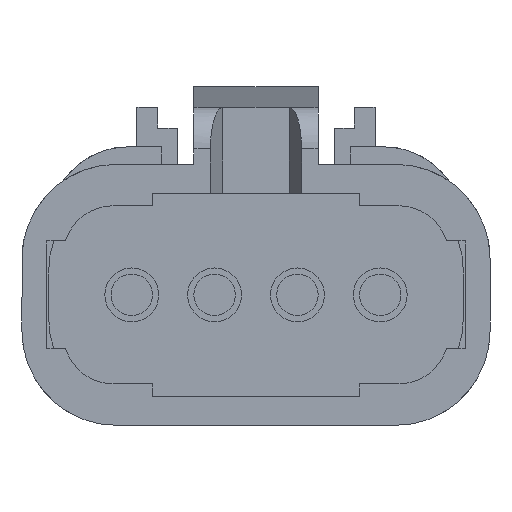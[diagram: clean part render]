
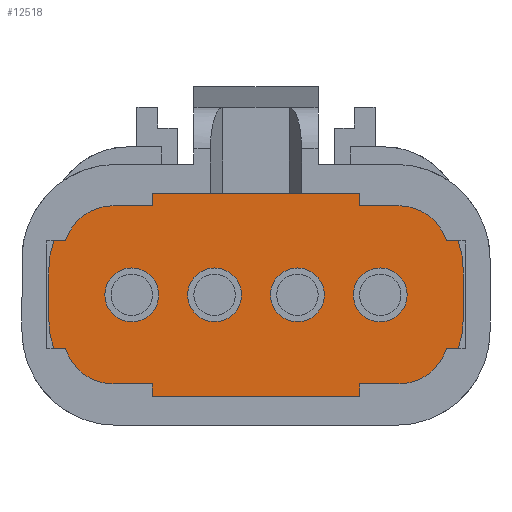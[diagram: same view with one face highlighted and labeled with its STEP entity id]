
A CAD part, front view. The second image highlights one B-rep face of the part: STEP entity #12518.
In plain terms, the highlighted planar face has unit normal (0, -1, 0).
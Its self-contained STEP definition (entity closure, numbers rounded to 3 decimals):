
#31 = CARTESIAN_POINT ( 'NONE',  ( 9.277, 0.032, 11.722 ) ) ;
#158 = DIRECTION ( 'NONE',  ( 0., -1., 0. ) ) ;
#267 = EDGE_CURVE ( 'NONE', #3505, #3678, #8905, .T. ) ;
#401 = DIRECTION ( 'NONE',  ( 0., 1., 0. ) ) ;
#629 = CIRCLE ( 'NONE', #10572, 0.65 ) ;
#683 = DIRECTION ( 'NONE',  ( 0., 0., 1. ) ) ;
#842 = EDGE_CURVE ( 'NONE', #3943, #9786, #10768, .T. ) ;
#934 = DIRECTION ( 'NONE',  ( -1., 0., 0. ) ) ;
#954 = CARTESIAN_POINT ( 'NONE',  ( 7.477, 0.032, 9.922 ) ) ;
#969 = LINE ( 'NONE', #7506, #8911 ) ;
#1073 = ORIENTED_EDGE ( 'NONE', *, *, #6733, .F. ) ;
#1563 = CARTESIAN_POINT ( 'NONE',  ( 3.927, 0.032, 12.372 ) ) ;
#1584 = CARTESIAN_POINT ( 'NONE',  ( -0.723, 0.032, 13.022 ) ) ;
#1592 = LINE ( 'NONE', #7227, #12161 ) ;
#1626 = FACE_OUTER_BOUND ( 'NONE', #8329, .T. ) ;
#1644 = CARTESIAN_POINT ( 'NONE',  ( 4.627, 0.032, 12.372 ) ) ;
#1683 = CARTESIAN_POINT ( 'NONE',  ( 1.077, 0.032, 13.022 ) ) ;
#1760 = CARTESIAN_POINT ( 'NONE',  ( 9.277, 0.032, 13.022 ) ) ;
#1831 = AXIS2_PLACEMENT_3D ( 'NONE', #9878, #13264, #3116 ) ;
#1903 = CARTESIAN_POINT ( 'NONE',  ( 0.627, 0.032, 12.372 ) ) ;
#1943 = CIRCLE ( 'NONE', #8327, 0.65 ) ;
#2380 = DIRECTION ( 'NONE',  ( -1., 0., 0. ) ) ;
#2409 = CARTESIAN_POINT ( 'NONE',  ( 7.277, 0.032, 12.372 ) ) ;
#2475 = EDGE_CURVE ( 'NONE', #8021, #3505, #8771, .T. ) ;
#2527 = EDGE_CURVE ( 'NONE', #9786, #3943, #1943, .T. ) ;
#2537 = CARTESIAN_POINT ( 'NONE',  ( 1.277, 0.032, 12.372 ) ) ;
#2554 = DIRECTION ( 'NONE',  ( -1., 0., 0. ) ) ;
#2583 = ORIENTED_EDGE ( 'NONE', *, *, #10625, .F. ) ;
#2644 = DIRECTION ( 'NONE',  ( -1., 0., 0. ) ) ;
#2749 = AXIS2_PLACEMENT_3D ( 'NONE', #13836, #8362, #7032 ) ;
#2914 = EDGE_CURVE ( 'NONE', #12138, #14171, #9163, .T. ) ;
#3116 = DIRECTION ( 'NONE',  ( -1., 0., 0. ) ) ;
#3173 = EDGE_CURVE ( 'NONE', #10151, #12673, #629, .T. ) ;
#3254 = AXIS2_PLACEMENT_3D ( 'NONE', #13728, #158, #13521 ) ;
#3291 = DIRECTION ( 'NONE',  ( 0., 0., -1. ) ) ;
#3296 = ORIENTED_EDGE ( 'NONE', *, *, #8671, .F. ) ;
#3456 = EDGE_CURVE ( 'NONE', #5921, #8046, #9171, .T. ) ;
#3505 = VERTEX_POINT ( 'NONE', #1584 ) ;
#3531 = DIRECTION ( 'NONE',  ( 1., 0., 0. ) ) ;
#3569 = DIRECTION ( 'NONE',  ( 0., -1., 0. ) ) ;
#3678 = VERTEX_POINT ( 'NONE', #6551 ) ;
#3943 = VERTEX_POINT ( 'NONE', #1563 ) ;
#4055 = VECTOR ( 'NONE', #683, 1000. ) ;
#4157 = FACE_BOUND ( 'NONE', #13364, .T. ) ;
#4186 = DIRECTION ( 'NONE',  ( 0., 1., 0. ) ) ;
#4331 = ORIENTED_EDGE ( 'NONE', *, *, #267, .F. ) ;
#4480 = CARTESIAN_POINT ( 'NONE',  ( 9.277, 0.032, 11.722 ) ) ;
#4681 = VERTEX_POINT ( 'NONE', #954 ) ;
#4792 = DIRECTION ( 'NONE',  ( 0., -1., 0. ) ) ;
#5004 = CARTESIAN_POINT ( 'NONE',  ( 7.477, 0.032, 11.722 ) ) ;
#5067 = ORIENTED_EDGE ( 'NONE', *, *, #2914, .F. ) ;
#5272 = EDGE_CURVE ( 'NONE', #4681, #8836, #969, .T. ) ;
#5325 = ORIENTED_EDGE ( 'NONE', *, *, #9541, .F. ) ;
#5363 = CIRCLE ( 'NONE', #2749, 0.65 ) ;
#5431 = CARTESIAN_POINT ( 'NONE',  ( 3.277, 0.032, 12.372 ) ) ;
#5501 = CARTESIAN_POINT ( 'NONE',  ( -0.723, 0.032, 11.722 ) ) ;
#5554 = EDGE_CURVE ( 'NONE', #14171, #12138, #5363, .T. ) ;
#5921 = VERTEX_POINT ( 'NONE', #11605 ) ;
#6033 = CARTESIAN_POINT ( 'NONE',  ( 1.927, 0.032, 12.372 ) ) ;
#6052 = AXIS2_PLACEMENT_3D ( 'NONE', #14604, #4186, #8924 ) ;
#6108 = CARTESIAN_POINT ( 'NONE',  ( 7.477, 0.032, 14.822 ) ) ;
#6206 = DIRECTION ( 'NONE',  ( 0., 1., 0. ) ) ;
#6244 = CIRCLE ( 'NONE', #9099, 0.65 ) ;
#6374 = FACE_BOUND ( 'NONE', #11573, .T. ) ;
#6500 = ORIENTED_EDGE ( 'NONE', *, *, #5272, .F. ) ;
#6551 = CARTESIAN_POINT ( 'NONE',  ( 1.077, 0.032, 14.822 ) ) ;
#6733 = EDGE_CURVE ( 'NONE', #8046, #5921, #6244, .T. ) ;
#6874 = AXIS2_PLACEMENT_3D ( 'NONE', #5004, #401, #14109 ) ;
#6899 = CARTESIAN_POINT ( 'NONE',  ( 3.277, 0.032, 12.372 ) ) ;
#6952 = CARTESIAN_POINT ( 'NONE',  ( 1.277, 0.032, 12.372 ) ) ;
#7032 = DIRECTION ( 'NONE',  ( -1., 0., 0. ) ) ;
#7153 = EDGE_CURVE ( 'NONE', #12673, #10151, #13356, .T. ) ;
#7222 = ORIENTED_EDGE ( 'NONE', *, *, #2527, .F. ) ;
#7227 = CARTESIAN_POINT ( 'NONE',  ( 7.477, 0.032, 14.822 ) ) ;
#7506 = CARTESIAN_POINT ( 'NONE',  ( 7.477, 0.032, 9.922 ) ) ;
#7743 = DIRECTION ( 'NONE',  ( -1., 0., 0. ) ) ;
#8021 = VERTEX_POINT ( 'NONE', #12366 ) ;
#8046 = VERTEX_POINT ( 'NONE', #12517 ) ;
#8293 = CIRCLE ( 'NONE', #10910, 1.8 ) ;
#8327 = AXIS2_PLACEMENT_3D ( 'NONE', #5431, #9967, #7743 ) ;
#8329 = EDGE_LOOP ( 'NONE', ( #3296, #6500, #12049, #2583, #5325, #14447, #4331, #14255 ) ) ;
#8362 = DIRECTION ( 'NONE',  ( 0., -1., 0. ) ) ;
#8407 = ORIENTED_EDGE ( 'NONE', *, *, #7153, .F. ) ;
#8579 = EDGE_LOOP ( 'NONE', ( #9759, #1073 ) ) ;
#8671 = EDGE_CURVE ( 'NONE', #8836, #8021, #12453, .T. ) ;
#8740 = DIRECTION ( 'NONE',  ( 0., 1., 0. ) ) ;
#8771 = LINE ( 'NONE', #5501, #4055 ) ;
#8836 = VERTEX_POINT ( 'NONE', #13852 ) ;
#8905 = CIRCLE ( 'NONE', #14339, 1.8 ) ;
#8911 = VECTOR ( 'NONE', #14444, 1000. ) ;
#8924 = DIRECTION ( 'NONE',  ( 1., 0., 0. ) ) ;
#9099 = AXIS2_PLACEMENT_3D ( 'NONE', #2409, #10275, #2554 ) ;
#9163 = CIRCLE ( 'NONE', #1831, 0.65 ) ;
#9171 = CIRCLE ( 'NONE', #3254, 0.65 ) ;
#9366 = DIRECTION ( 'NONE',  ( 0., -1., 0. ) ) ;
#9523 = DIRECTION ( 'NONE',  ( 1., 0., 0. ) ) ;
#9541 = EDGE_CURVE ( 'NONE', #14196, #11252, #8293, .T. ) ;
#9659 = VERTEX_POINT ( 'NONE', #31 ) ;
#9723 = EDGE_CURVE ( 'NONE', #9659, #4681, #12090, .T. ) ;
#9759 = ORIENTED_EDGE ( 'NONE', *, *, #3456, .F. ) ;
#9786 = VERTEX_POINT ( 'NONE', #12933 ) ;
#9878 = CARTESIAN_POINT ( 'NONE',  ( 5.277, 0.032, 12.372 ) ) ;
#9967 = DIRECTION ( 'NONE',  ( 0., -1., 0. ) ) ;
#10151 = VERTEX_POINT ( 'NONE', #1903 ) ;
#10275 = DIRECTION ( 'NONE',  ( 0., -1., 0. ) ) ;
#10572 = AXIS2_PLACEMENT_3D ( 'NONE', #6952, #4792, #2644 ) ;
#10625 = EDGE_CURVE ( 'NONE', #11252, #9659, #11300, .T. ) ;
#10768 = CIRCLE ( 'NONE', #13143, 0.65 ) ;
#10897 = FACE_BOUND ( 'NONE', #8579, .T. ) ;
#10910 = AXIS2_PLACEMENT_3D ( 'NONE', #14358, #8740, #12131 ) ;
#10948 = EDGE_LOOP ( 'NONE', ( #7222, #13594 ) ) ;
#10969 = CARTESIAN_POINT ( 'NONE',  ( 1.077, 0.032, 11.722 ) ) ;
#11252 = VERTEX_POINT ( 'NONE', #1760 ) ;
#11300 = LINE ( 'NONE', #4480, #12545 ) ;
#11474 = EDGE_CURVE ( 'NONE', #3678, #14196, #1592, .T. ) ;
#11573 = EDGE_LOOP ( 'NONE', ( #5067, #12139 ) ) ;
#11605 = CARTESIAN_POINT ( 'NONE',  ( 6.627, 0.032, 12.372 ) ) ;
#12049 = ORIENTED_EDGE ( 'NONE', *, *, #9723, .F. ) ;
#12090 = CIRCLE ( 'NONE', #6874, 1.8 ) ;
#12131 = DIRECTION ( 'NONE',  ( 1., 0., 0. ) ) ;
#12138 = VERTEX_POINT ( 'NONE', #1644 ) ;
#12139 = ORIENTED_EDGE ( 'NONE', *, *, #5554, .F. ) ;
#12161 = VECTOR ( 'NONE', #9523, 1000. ) ;
#12175 = AXIS2_PLACEMENT_3D ( 'NONE', #2537, #9366, #12481 ) ;
#12366 = CARTESIAN_POINT ( 'NONE',  ( -0.723, 0.032, 11.722 ) ) ;
#12453 = CIRCLE ( 'NONE', #6052, 1.8 ) ;
#12481 = DIRECTION ( 'NONE',  ( -1., 0., 0. ) ) ;
#12517 = CARTESIAN_POINT ( 'NONE',  ( 7.927, 0.032, 12.372 ) ) ;
#12518 = ADVANCED_FACE ( 'NONE', ( #4157, #14065, #6374, #10897, #1626 ), #12803, .F. ) ;
#12545 = VECTOR ( 'NONE', #3291, 1000. ) ;
#12673 = VERTEX_POINT ( 'NONE', #6033 ) ;
#12800 = ORIENTED_EDGE ( 'NONE', *, *, #3173, .F. ) ;
#12803 = PLANE ( 'NONE',  #13609 ) ;
#12933 = CARTESIAN_POINT ( 'NONE',  ( 2.627, 0.032, 12.372 ) ) ;
#12998 = CARTESIAN_POINT ( 'NONE',  ( 5.927, 0.032, 12.372 ) ) ;
#13143 = AXIS2_PLACEMENT_3D ( 'NONE', #6899, #3569, #2380 ) ;
#13264 = DIRECTION ( 'NONE',  ( 0., -1., 0. ) ) ;
#13356 = CIRCLE ( 'NONE', #12175, 0.65 ) ;
#13364 = EDGE_LOOP ( 'NONE', ( #12800, #8407 ) ) ;
#13521 = DIRECTION ( 'NONE',  ( -1., 0., 0. ) ) ;
#13594 = ORIENTED_EDGE ( 'NONE', *, *, #842, .F. ) ;
#13609 = AXIS2_PLACEMENT_3D ( 'NONE', #10969, #14632, #3531 ) ;
#13728 = CARTESIAN_POINT ( 'NONE',  ( 7.277, 0.032, 12.372 ) ) ;
#13836 = CARTESIAN_POINT ( 'NONE',  ( 5.277, 0.032, 12.372 ) ) ;
#13852 = CARTESIAN_POINT ( 'NONE',  ( 1.077, 0.032, 9.922 ) ) ;
#14065 = FACE_BOUND ( 'NONE', #10948, .T. ) ;
#14109 = DIRECTION ( 'NONE',  ( -1., 0., 0. ) ) ;
#14171 = VERTEX_POINT ( 'NONE', #12998 ) ;
#14196 = VERTEX_POINT ( 'NONE', #6108 ) ;
#14255 = ORIENTED_EDGE ( 'NONE', *, *, #2475, .F. ) ;
#14339 = AXIS2_PLACEMENT_3D ( 'NONE', #1683, #6206, #934 ) ;
#14358 = CARTESIAN_POINT ( 'NONE',  ( 7.477, 0.032, 13.022 ) ) ;
#14444 = DIRECTION ( 'NONE',  ( -1., 0., 0. ) ) ;
#14447 = ORIENTED_EDGE ( 'NONE', *, *, #11474, .F. ) ;
#14604 = CARTESIAN_POINT ( 'NONE',  ( 1.077, 0.032, 11.722 ) ) ;
#14632 = DIRECTION ( 'NONE',  ( 0., 1., 0. ) ) ;
